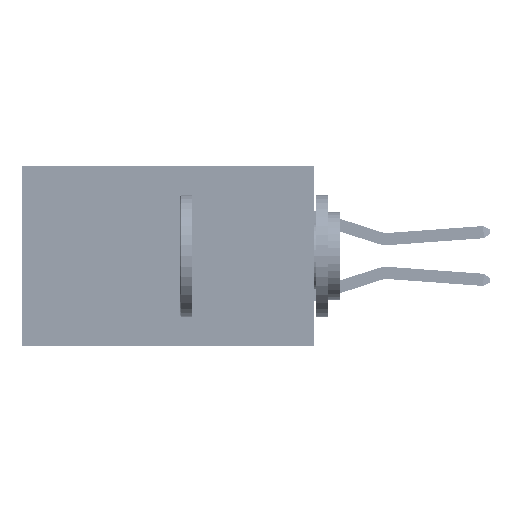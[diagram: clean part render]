
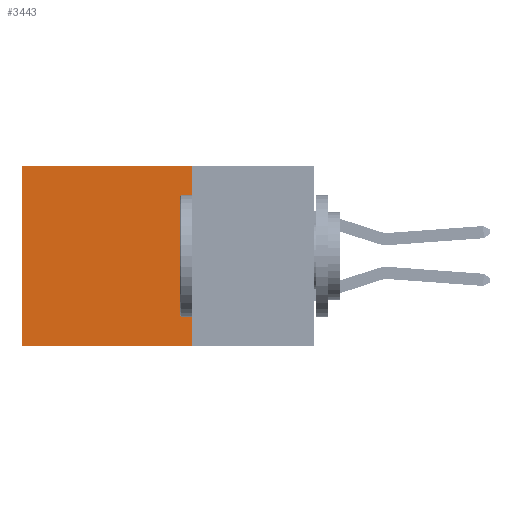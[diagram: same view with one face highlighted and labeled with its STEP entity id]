
A CAD part, left-side view. The second image highlights one B-rep face of the part: STEP entity #3443.
In plain terms, the highlighted planar face has unit normal (-1, 0, 0).
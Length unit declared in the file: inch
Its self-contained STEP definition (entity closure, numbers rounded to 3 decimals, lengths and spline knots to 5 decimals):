
#470 = CARTESIAN_POINT ( 'NONE',  ( 0.2875, 0.25, -0.37 ) ) ;
#2455 = EDGE_CURVE ( 'NONE', #3353, #41216, #45226, .T. ) ;
#3293 = VERTEX_POINT ( 'NONE', #12975 ) ;
#3353 = VERTEX_POINT ( 'NONE', #35611 ) ;
#3443 = ADVANCED_FACE ( 'NONE', ( #41598 ), #47426, .F. ) ;
#3684 = DIRECTION ( 'NONE',  ( 0., 1., 0. ) ) ;
#5515 = ORIENTED_EDGE ( 'NONE', *, *, #2455, .F. ) ;
#6224 = DIRECTION ( 'NONE',  ( 0., 0., -1. ) ) ;
#8442 = CARTESIAN_POINT ( 'NONE',  ( 0.2875, 0.25, 0. ) ) ;
#8513 = VERTEX_POINT ( 'NONE', #9694 ) ;
#9694 = CARTESIAN_POINT ( 'NONE',  ( 0.2875, 0.6, -0.37 ) ) ;
#11160 = VECTOR ( 'NONE', #3684, 39.37008 ) ;
#11835 = AXIS2_PLACEMENT_3D ( 'NONE', #24897, #28682, #6224 ) ;
#12975 = CARTESIAN_POINT ( 'NONE',  ( 0.2875, 0.6, 0. ) ) ;
#16121 = ORIENTED_EDGE ( 'NONE', *, *, #18378, .T. ) ;
#16446 = VECTOR ( 'NONE', #39513, 39.37008 ) ;
#17600 = VECTOR ( 'NONE', #23313, 39.37008 ) ;
#17743 = EDGE_LOOP ( 'NONE', ( #16121, #26579, #5515, #43590 ) ) ;
#18378 = EDGE_CURVE ( 'NONE', #3293, #8513, #18791, .T. ) ;
#18791 = LINE ( 'NONE', #20580, #16446 ) ;
#19264 = VECTOR ( 'NONE', #45489, 39.37008 ) ;
#20436 = LINE ( 'NONE', #470, #19264 ) ;
#20580 = CARTESIAN_POINT ( 'NONE',  ( 0.2875, 0.6, 0. ) ) ;
#21114 = LINE ( 'NONE', #33560, #11160 ) ;
#23313 = DIRECTION ( 'NONE',  ( 0., 0., -1. ) ) ;
#24897 = CARTESIAN_POINT ( 'NONE',  ( 0.2875, 0.25, 0. ) ) ;
#26579 = ORIENTED_EDGE ( 'NONE', *, *, #40307, .F. ) ;
#28682 = DIRECTION ( 'NONE',  ( 1., 0., 0. ) ) ;
#33560 = CARTESIAN_POINT ( 'NONE',  ( 0.2875, 0.25, 0. ) ) ;
#35611 = CARTESIAN_POINT ( 'NONE',  ( 0.2875, 0.25, 0. ) ) ;
#39513 = DIRECTION ( 'NONE',  ( 0., 0., -1. ) ) ;
#40307 = EDGE_CURVE ( 'NONE', #41216, #8513, #20436, .T. ) ;
#41216 = VERTEX_POINT ( 'NONE', #42035 ) ;
#41598 = FACE_OUTER_BOUND ( 'NONE', #17743, .T. ) ;
#42035 = CARTESIAN_POINT ( 'NONE',  ( 0.2875, 0.25, -0.37 ) ) ;
#43590 = ORIENTED_EDGE ( 'NONE', *, *, #45131, .T. ) ;
#45131 = EDGE_CURVE ( 'NONE', #3353, #3293, #21114, .T. ) ;
#45226 = LINE ( 'NONE', #8442, #17600 ) ;
#45489 = DIRECTION ( 'NONE',  ( 0., 1., 0. ) ) ;
#47426 = PLANE ( 'NONE',  #11835 ) ;
